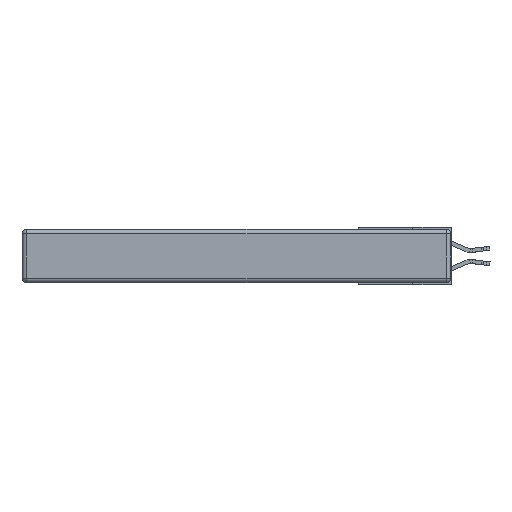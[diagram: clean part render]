
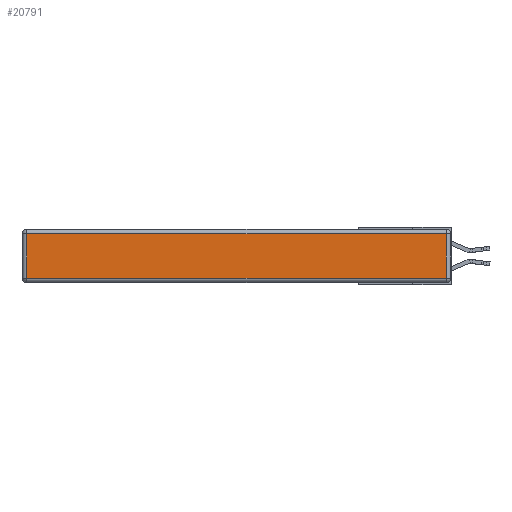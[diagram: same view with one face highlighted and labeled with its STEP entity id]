
A CAD part, left-side view. The second image highlights one B-rep face of the part: STEP entity #20791.
In plain terms, the highlighted planar face has unit normal (-1, 0, 0).
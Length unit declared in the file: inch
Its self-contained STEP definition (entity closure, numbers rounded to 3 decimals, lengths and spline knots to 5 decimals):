
#1153 = DIRECTION ( 'NONE',  ( 0., 0., 1. ) ) ;
#1438 = ORIENTED_EDGE ( 'NONE', *, *, #11854, .T. ) ;
#2143 = VERTEX_POINT ( 'NONE', #10920 ) ;
#2675 = VERTEX_POINT ( 'NONE', #26270 ) ;
#3952 = LINE ( 'NONE', #10065, #27250 ) ;
#6430 = DIRECTION ( 'NONE',  ( 0., 0., 1. ) ) ;
#6884 = AXIS2_PLACEMENT_3D ( 'NONE', #9095, #20007, #6430 ) ;
#7832 = CARTESIAN_POINT ( 'NONE',  ( 0., 0.03, -0.313 ) ) ;
#7962 = EDGE_CURVE ( 'NONE', #2143, #2675, #15013, .T. ) ;
#8110 = ORIENTED_EDGE ( 'NONE', *, *, #28282, .T. ) ;
#9095 = CARTESIAN_POINT ( 'NONE',  ( 0., 0., -0.343 ) ) ;
#10065 = CARTESIAN_POINT ( 'NONE',  ( 0., 2.75, -0.03 ) ) ;
#10920 = CARTESIAN_POINT ( 'NONE',  ( 0., 2.72, -0.03 ) ) ;
#11854 = EDGE_CURVE ( 'NONE', #2675, #33254, #30253, .T. ) ;
#11887 = EDGE_LOOP ( 'NONE', ( #1438, #15714, #8110, #31697 ) ) ;
#12215 = EDGE_CURVE ( 'NONE', #33254, #32430, #15998, .T. ) ;
#14504 = CARTESIAN_POINT ( 'NONE',  ( 0., 2.72, -0.343 ) ) ;
#14735 = DIRECTION ( 'NONE',  ( 0., 0., -1. ) ) ;
#15013 = LINE ( 'NONE', #14504, #32669 ) ;
#15542 = DIRECTION ( 'NONE',  ( 0., 1., 0. ) ) ;
#15714 = ORIENTED_EDGE ( 'NONE', *, *, #12215, .T. ) ;
#15998 = LINE ( 'NONE', #25710, #19018 ) ;
#19018 = VECTOR ( 'NONE', #1153, 39.37008 ) ;
#20007 = DIRECTION ( 'NONE',  ( -1., 0., 0. ) ) ;
#20791 = ADVANCED_FACE ( 'NONE', ( #31896 ), #34080, .T. ) ;
#25710 = CARTESIAN_POINT ( 'NONE',  ( 0., 0.03, -0.343 ) ) ;
#26270 = CARTESIAN_POINT ( 'NONE',  ( 0., 2.72, -0.313 ) ) ;
#27250 = VECTOR ( 'NONE', #15542, 39.37008 ) ;
#28282 = EDGE_CURVE ( 'NONE', #32430, #2143, #3952, .T. ) ;
#29628 = DIRECTION ( 'NONE',  ( 0., -1., 0. ) ) ;
#29757 = CARTESIAN_POINT ( 'NONE',  ( 0., 0., -0.313 ) ) ;
#30253 = LINE ( 'NONE', #29757, #31585 ) ;
#31585 = VECTOR ( 'NONE', #29628, 39.37008 ) ;
#31697 = ORIENTED_EDGE ( 'NONE', *, *, #7962, .T. ) ;
#31756 = CARTESIAN_POINT ( 'NONE',  ( 0., 0.03, -0.03 ) ) ;
#31896 = FACE_OUTER_BOUND ( 'NONE', #11887, .T. ) ;
#32430 = VERTEX_POINT ( 'NONE', #31756 ) ;
#32669 = VECTOR ( 'NONE', #14735, 39.37008 ) ;
#33254 = VERTEX_POINT ( 'NONE', #7832 ) ;
#34080 = PLANE ( 'NONE',  #6884 ) ;
